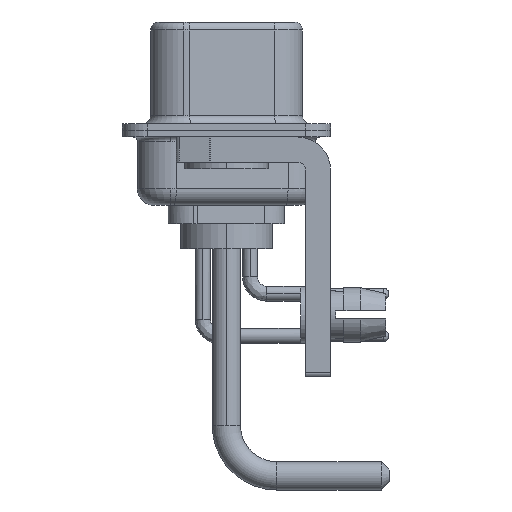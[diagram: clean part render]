
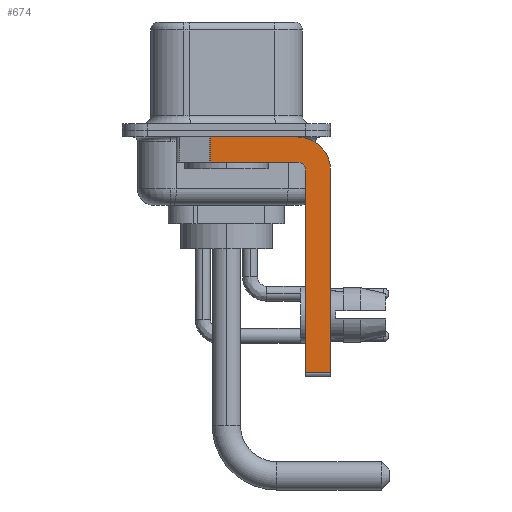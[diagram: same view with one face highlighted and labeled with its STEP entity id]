
A CAD part, left-side view. The second image highlights one B-rep face of the part: STEP entity #674.
In plain terms, the highlighted planar face has unit normal (-1, 0, 0).
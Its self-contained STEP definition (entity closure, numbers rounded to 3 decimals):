
#60 = CARTESIAN_POINT ( 'NONE',  ( -2.9, -4.25, -14.55 ) ) ;
#124 = CIRCLE ( 'NONE', #6831, 2. ) ;
#454 = ORIENTED_EDGE ( 'NONE', *, *, #13899, .F. ) ;
#674 = ADVANCED_FACE ( 'NONE', ( #2421 ), #2550, .F. ) ;
#1309 = EDGE_LOOP ( 'NONE', ( #9149, #6231, #11036, #12702, #454, #4896, #18430, #17103 ) ) ;
#2421 = FACE_OUTER_BOUND ( 'NONE', #1309, .T. ) ;
#2550 = PLANE ( 'NONE',  #7507 ) ;
#3259 = EDGE_CURVE ( 'NONE', #13985, #25594, #11897, .T. ) ;
#4159 = DIRECTION ( 'NONE',  ( 1., 0., 0. ) ) ;
#4245 = LINE ( 'NONE', #16593, #14706 ) ;
#4645 = DIRECTION ( 'NONE',  ( 0., 0., 1. ) ) ;
#4896 = ORIENTED_EDGE ( 'NONE', *, *, #9058, .T. ) ;
#5017 = EDGE_CURVE ( 'NONE', #12750, #17620, #12525, .T. ) ;
#5080 = CARTESIAN_POINT ( 'NONE',  ( -2.9, -6.25, -2.4 ) ) ;
#5497 = VECTOR ( 'NONE', #4645, 1000. ) ;
#5988 = DIRECTION ( 'NONE',  ( -1., 0., 0. ) ) ;
#6212 = LINE ( 'NONE', #6335, #5497 ) ;
#6231 = ORIENTED_EDGE ( 'NONE', *, *, #5017, .T. ) ;
#6255 = VERTEX_POINT ( 'NONE', #23971 ) ;
#6256 = DIRECTION ( 'NONE',  ( 0., 1., 0. ) ) ;
#6335 = CARTESIAN_POINT ( 'NONE',  ( -2.9, -4.75, -14.8 ) ) ;
#6595 = DIRECTION ( 'NONE',  ( 0., -1., 0. ) ) ;
#6637 = VERTEX_POINT ( 'NONE', #5080 ) ;
#6831 = AXIS2_PLACEMENT_3D ( 'NONE', #14001, #4159, #18206 ) ;
#6994 = CARTESIAN_POINT ( 'NONE',  ( -2.9, 0.978, -1.9 ) ) ;
#7507 = AXIS2_PLACEMENT_3D ( 'NONE', #8721, #24867, #16616 ) ;
#7906 = CARTESIAN_POINT ( 'NONE',  ( -2.9, -4.25, -1.9 ) ) ;
#8221 = CARTESIAN_POINT ( 'NONE',  ( -2.9, -4.25, -2.4 ) ) ;
#8568 = CARTESIAN_POINT ( 'NONE',  ( -2.9, -4.75, -2.4 ) ) ;
#8721 = CARTESIAN_POINT ( 'NONE',  ( -2.9, -4.25, -2.4 ) ) ;
#9058 = EDGE_CURVE ( 'NONE', #6255, #9964, #10047, .T. ) ;
#9117 = CARTESIAN_POINT ( 'NONE',  ( -2.9, -6.25, -2.4 ) ) ;
#9149 = ORIENTED_EDGE ( 'NONE', *, *, #13892, .F. ) ;
#9964 = VERTEX_POINT ( 'NONE', #15875 ) ;
#10047 = LINE ( 'NONE', #60, #25474 ) ;
#10762 = EDGE_CURVE ( 'NONE', #6637, #9964, #15279, .T. ) ;
#11036 = ORIENTED_EDGE ( 'NONE', *, *, #24664, .F. ) ;
#11897 = CIRCLE ( 'NONE', #15241, 0.5 ) ;
#12525 = LINE ( 'NONE', #24727, #12697 ) ;
#12650 = VERTEX_POINT ( 'NONE', #15124 ) ;
#12697 = VECTOR ( 'NONE', #24606, 1000. ) ;
#12702 = ORIENTED_EDGE ( 'NONE', *, *, #3259, .F. ) ;
#12750 = VERTEX_POINT ( 'NONE', #19997 ) ;
#13892 = EDGE_CURVE ( 'NONE', #12750, #12650, #4245, .T. ) ;
#13899 = EDGE_CURVE ( 'NONE', #6255, #13985, #6212, .T. ) ;
#13985 = VERTEX_POINT ( 'NONE', #8568 ) ;
#14001 = CARTESIAN_POINT ( 'NONE',  ( -2.9, -4.25, -2.4 ) ) ;
#14706 = VECTOR ( 'NONE', #6595, 1000. ) ;
#14865 = VECTOR ( 'NONE', #6256, 1000. ) ;
#15124 = CARTESIAN_POINT ( 'NONE',  ( -2.9, -4.25, -0.4 ) ) ;
#15241 = AXIS2_PLACEMENT_3D ( 'NONE', #8221, #5988, #21996 ) ;
#15279 = LINE ( 'NONE', #9117, #17946 ) ;
#15875 = CARTESIAN_POINT ( 'NONE',  ( -2.9, -6.25, -14.55 ) ) ;
#16593 = CARTESIAN_POINT ( 'NONE',  ( -2.9, 3., -0.4 ) ) ;
#16616 = DIRECTION ( 'NONE',  ( 0., 0., -1. ) ) ;
#17103 = ORIENTED_EDGE ( 'NONE', *, *, #23336, .F. ) ;
#17620 = VERTEX_POINT ( 'NONE', #6994 ) ;
#17946 = VECTOR ( 'NONE', #21061, 1000. ) ;
#18206 = DIRECTION ( 'NONE',  ( 0., 0., -1. ) ) ;
#18430 = ORIENTED_EDGE ( 'NONE', *, *, #10762, .F. ) ;
#19997 = CARTESIAN_POINT ( 'NONE',  ( -2.9, 0.978, -0.4 ) ) ;
#20178 = DIRECTION ( 'NONE',  ( 0., -1., 0. ) ) ;
#21061 = DIRECTION ( 'NONE',  ( 0., 0., -1. ) ) ;
#21996 = DIRECTION ( 'NONE',  ( 0., 0., 1. ) ) ;
#23336 = EDGE_CURVE ( 'NONE', #12650, #6637, #124, .T. ) ;
#23969 = LINE ( 'NONE', #24101, #14865 ) ;
#23971 = CARTESIAN_POINT ( 'NONE',  ( -2.9, -4.75, -14.55 ) ) ;
#24101 = CARTESIAN_POINT ( 'NONE',  ( -2.9, -4.25, -1.9 ) ) ;
#24606 = DIRECTION ( 'NONE',  ( 0., 0., -1. ) ) ;
#24664 = EDGE_CURVE ( 'NONE', #25594, #17620, #23969, .T. ) ;
#24727 = CARTESIAN_POINT ( 'NONE',  ( -2.9, 0.978, -1.9 ) ) ;
#24867 = DIRECTION ( 'NONE',  ( 1., 0., 0. ) ) ;
#25474 = VECTOR ( 'NONE', #20178, 1000. ) ;
#25594 = VERTEX_POINT ( 'NONE', #7906 ) ;
